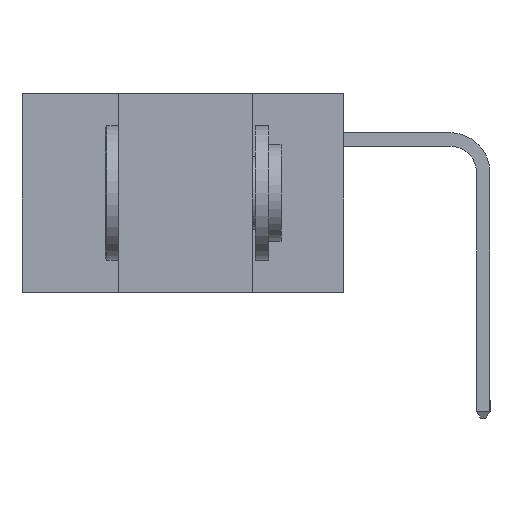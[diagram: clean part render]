
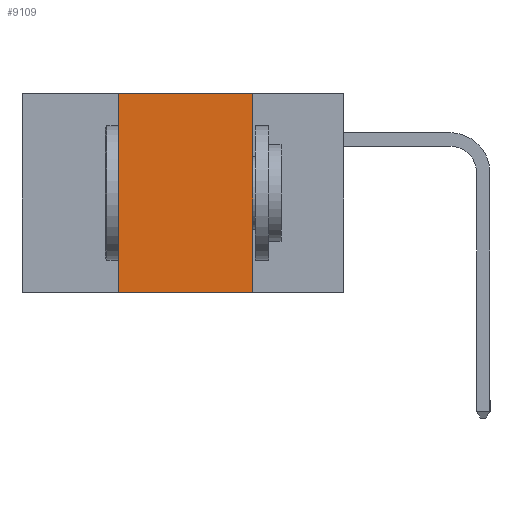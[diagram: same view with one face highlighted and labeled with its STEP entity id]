
A CAD part, left-side view. The second image highlights one B-rep face of the part: STEP entity #9109.
In plain terms, the highlighted planar face has unit normal (-1, 0, 0).
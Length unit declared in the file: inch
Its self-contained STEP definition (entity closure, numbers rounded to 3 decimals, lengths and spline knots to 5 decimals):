
#397 = VECTOR ( 'NONE', #8075, 39.37008 ) ;
#433 = FACE_OUTER_BOUND ( 'NONE', #12469, .T. ) ;
#1196 = EDGE_CURVE ( 'NONE', #17673, #16906, #5758, .T. ) ;
#2514 = EDGE_CURVE ( 'NONE', #16906, #3580, #10367, .T. ) ;
#3024 = DIRECTION ( 'NONE',  ( 0., 0., -1. ) ) ;
#3170 = CARTESIAN_POINT ( 'NONE',  ( 0., 0.17, -0.37 ) ) ;
#3580 = VERTEX_POINT ( 'NONE', #19457 ) ;
#5115 = VECTOR ( 'NONE', #13566, 39.37008 ) ;
#5758 = LINE ( 'NONE', #15129, #5115 ) ;
#6146 = CARTESIAN_POINT ( 'NONE',  ( 0., 0.17, 0. ) ) ;
#8017 = DIRECTION ( 'NONE',  ( 0., 0., -1. ) ) ;
#8029 = DIRECTION ( 'NONE',  ( 1., 0., 0. ) ) ;
#8075 = DIRECTION ( 'NONE',  ( 0., -1., 0. ) ) ;
#8088 = PLANE ( 'NONE',  #13210 ) ;
#8222 = CARTESIAN_POINT ( 'NONE',  ( 0., 0.6, 0. ) ) ;
#9109 = ADVANCED_FACE ( 'NONE', ( #433 ), #8088, .F. ) ;
#9750 = VECTOR ( 'NONE', #3024, 39.37008 ) ;
#10366 = CARTESIAN_POINT ( 'NONE',  ( 0., 0.42, -0.37 ) ) ;
#10367 = LINE ( 'NONE', #3170, #9750 ) ;
#10957 = LINE ( 'NONE', #13904, #397 ) ;
#12469 = EDGE_LOOP ( 'NONE', ( #16096, #16698, #21765, #22896 ) ) ;
#12681 = VECTOR ( 'NONE', #16215, 39.37008 ) ;
#13210 = AXIS2_PLACEMENT_3D ( 'NONE', #8222, #8029, #8017 ) ;
#13566 = DIRECTION ( 'NONE',  ( 0., -1., 0. ) ) ;
#13904 = CARTESIAN_POINT ( 'NONE',  ( 0., 0.6, -0.37 ) ) ;
#14359 = VERTEX_POINT ( 'NONE', #22891 ) ;
#15129 = CARTESIAN_POINT ( 'NONE',  ( 0., 0.6, 0. ) ) ;
#16096 = ORIENTED_EDGE ( 'NONE', *, *, #2514, .F. ) ;
#16215 = DIRECTION ( 'NONE',  ( 0., 0., 1. ) ) ;
#16698 = ORIENTED_EDGE ( 'NONE', *, *, #1196, .F. ) ;
#16906 = VERTEX_POINT ( 'NONE', #6146 ) ;
#17673 = VERTEX_POINT ( 'NONE', #21952 ) ;
#18387 = LINE ( 'NONE', #10366, #12681 ) ;
#18745 = EDGE_CURVE ( 'NONE', #14359, #3580, #10957, .T. ) ;
#19457 = CARTESIAN_POINT ( 'NONE',  ( 0., 0.17, -0.37 ) ) ;
#21327 = EDGE_CURVE ( 'NONE', #14359, #17673, #18387, .T. ) ;
#21765 = ORIENTED_EDGE ( 'NONE', *, *, #21327, .F. ) ;
#21952 = CARTESIAN_POINT ( 'NONE',  ( 0., 0.42, 0. ) ) ;
#22891 = CARTESIAN_POINT ( 'NONE',  ( 0., 0.42, -0.37 ) ) ;
#22896 = ORIENTED_EDGE ( 'NONE', *, *, #18745, .T. ) ;
